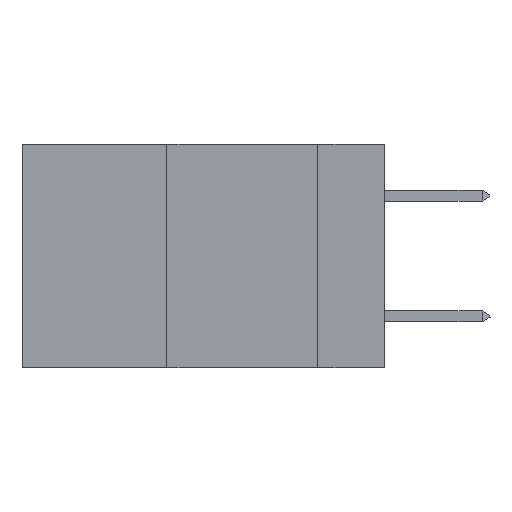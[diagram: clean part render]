
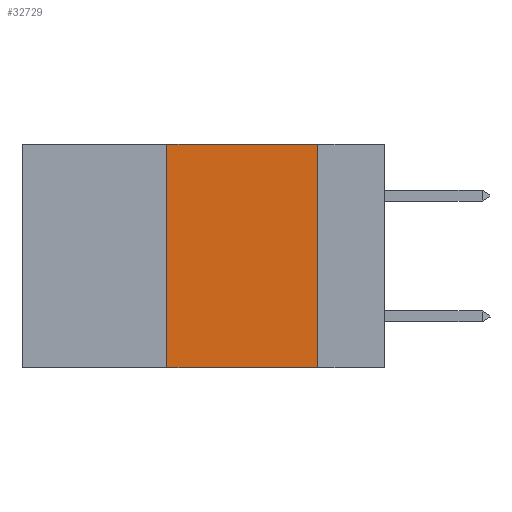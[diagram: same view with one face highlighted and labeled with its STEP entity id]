
A CAD part, left-side view. The second image highlights one B-rep face of the part: STEP entity #32729.
In plain terms, the highlighted planar face has unit normal (-1, 0, 0).
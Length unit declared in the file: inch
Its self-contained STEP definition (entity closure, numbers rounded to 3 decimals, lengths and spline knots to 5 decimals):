
#116 = VECTOR ( 'NONE', #6114, 39.37008 ) ;
#929 = CARTESIAN_POINT ( 'NONE',  ( 0., 0.36, -0.37 ) ) ;
#1027 = ORIENTED_EDGE ( 'NONE', *, *, #4583, .F. ) ;
#1336 = LINE ( 'NONE', #19264, #116 ) ;
#1347 = AXIS2_PLACEMENT_3D ( 'NONE', #10662, #29004, #31713 ) ;
#1709 = ORIENTED_EDGE ( 'NONE', *, *, #14666, .F. ) ;
#2546 = CARTESIAN_POINT ( 'NONE',  ( 0., 0.11, -0.37 ) ) ;
#3877 = LINE ( 'NONE', #24797, #26358 ) ;
#4232 = CARTESIAN_POINT ( 'NONE',  ( 0., 0.11, 0. ) ) ;
#4317 = VERTEX_POINT ( 'NONE', #929 ) ;
#4583 = EDGE_CURVE ( 'NONE', #29011, #32621, #3877, .T. ) ;
#5093 = ORIENTED_EDGE ( 'NONE', *, *, #14651, .F. ) ;
#5874 = EDGE_LOOP ( 'NONE', ( #1027, #5093, #1709, #32382 ) ) ;
#6114 = DIRECTION ( 'NONE',  ( 0., -1., 0. ) ) ;
#6349 = CARTESIAN_POINT ( 'NONE',  ( 0., 0.36, 0. ) ) ;
#7682 = CARTESIAN_POINT ( 'NONE',  ( 0., 0.6, -0.37 ) ) ;
#10662 = CARTESIAN_POINT ( 'NONE',  ( 0., 0.6, 0. ) ) ;
#12111 = VECTOR ( 'NONE', #23523, 39.37008 ) ;
#14651 = EDGE_CURVE ( 'NONE', #18677, #29011, #1336, .T. ) ;
#14666 = EDGE_CURVE ( 'NONE', #4317, #18677, #20212, .T. ) ;
#18677 = VERTEX_POINT ( 'NONE', #29640 ) ;
#19264 = CARTESIAN_POINT ( 'NONE',  ( 0., 0.6, 0. ) ) ;
#20212 = LINE ( 'NONE', #6349, #21026 ) ;
#21026 = VECTOR ( 'NONE', #32579, 39.37008 ) ;
#21250 = PLANE ( 'NONE',  #1347 ) ;
#21621 = FACE_OUTER_BOUND ( 'NONE', #5874, .T. ) ;
#22644 = LINE ( 'NONE', #7682, #12111 ) ;
#23523 = DIRECTION ( 'NONE',  ( 0., -1., 0. ) ) ;
#24797 = CARTESIAN_POINT ( 'NONE',  ( 0., 0.11, 0. ) ) ;
#26358 = VECTOR ( 'NONE', #30161, 39.37008 ) ;
#29004 = DIRECTION ( 'NONE',  ( 1., 0., 0. ) ) ;
#29011 = VERTEX_POINT ( 'NONE', #4232 ) ;
#29316 = EDGE_CURVE ( 'NONE', #4317, #32621, #22644, .T. ) ;
#29640 = CARTESIAN_POINT ( 'NONE',  ( 0., 0.36, 0. ) ) ;
#30161 = DIRECTION ( 'NONE',  ( 0., 0., -1. ) ) ;
#31713 = DIRECTION ( 'NONE',  ( 0., 0., -1. ) ) ;
#32382 = ORIENTED_EDGE ( 'NONE', *, *, #29316, .T. ) ;
#32579 = DIRECTION ( 'NONE',  ( 0., 0., 1. ) ) ;
#32621 = VERTEX_POINT ( 'NONE', #2546 ) ;
#32729 = ADVANCED_FACE ( 'NONE', ( #21621 ), #21250, .F. ) ;
